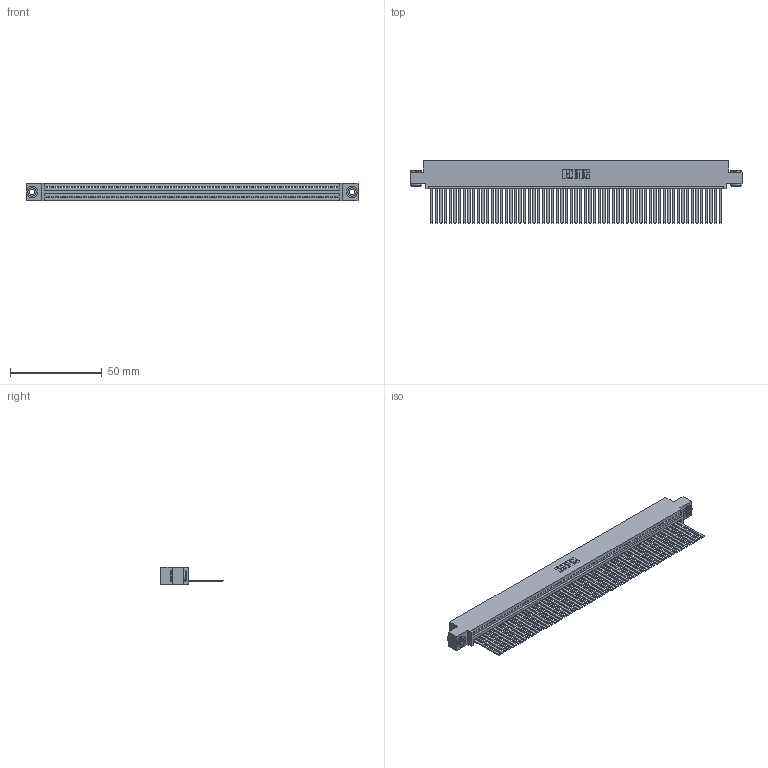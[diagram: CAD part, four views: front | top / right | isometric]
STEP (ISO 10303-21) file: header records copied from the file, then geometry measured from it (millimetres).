
FILE_DESCRIPTION (( 'STEP AP203' ), '1' );
FILE_NAME ('345-063-544-403.STEP', '2018-09-28T02:19:03', ( '' ), ( '' ), 'SwSTEP 2.0', 'SolidWorks 2016', '' );
FILE_SCHEMA (( 'CONFIG_CONTROL_DESIGN' ));
Length unit declared in the file: inch
Products named in the file (4): 345-292-001_345-293-144; 345-063-544-403; 345 Part_0.110 Offset - 0.156 Dia-TH; 345-250-002_345-250-002-102
Assembly tree (66 placements, depth 2):
  345-063-544-403
    345 Part_0.110 Offset - 0.156 Dia-TH
    345-292-001_345-293-144  x63
    345-250-002_345-250-002-102  x2
Bounding box: 181.23 x 33.96 x 9.4 mm (x, y, z)
Volume: 18061 mm3; surface area: 26773.6 mm2
Topology: 66 solids, 66 shells, 3444 faces, 10383 edges, 6834 vertices
Faces by surface type: plane 2362, cylinder 1074, cone 8
Entity records: 45186 total; most frequent: CARTESIAN_POINT 7804, ORIENTED_EDGE 7794, DIRECTION 6813, EDGE_CURVE 3897, LINE 3493, VECTOR 3493, VERTEX_POINT 2594, AXIS2_PLACEMENT_3D 1660
